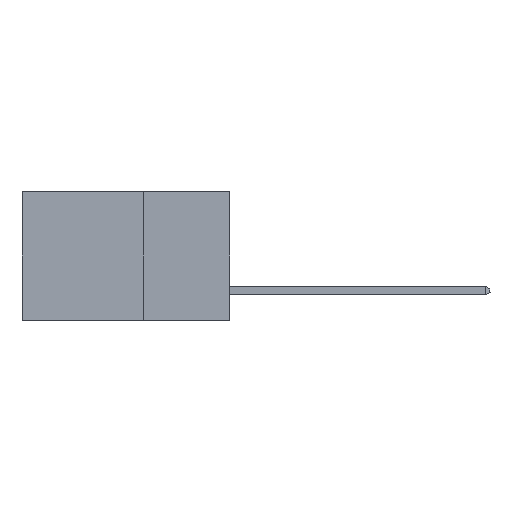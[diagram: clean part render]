
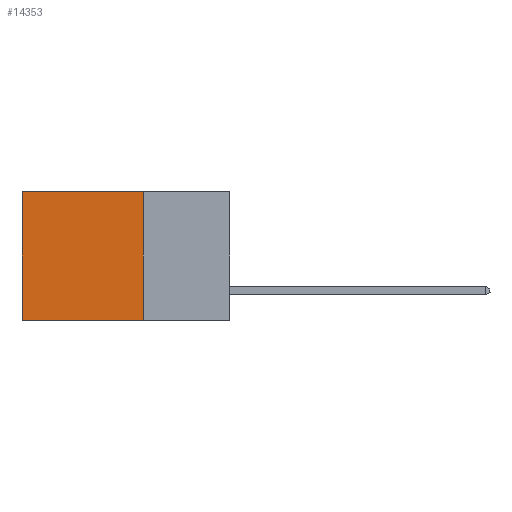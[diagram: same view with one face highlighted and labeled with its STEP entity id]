
A CAD part, left-side view. The second image highlights one B-rep face of the part: STEP entity #14353.
In plain terms, the highlighted planar face has unit normal (-1, 0, 0).
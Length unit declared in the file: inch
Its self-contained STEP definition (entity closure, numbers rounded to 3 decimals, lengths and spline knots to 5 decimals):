
#10 = EDGE_CURVE ( 'NONE', #11506, #3457, #2762, .T. ) ;
#201 = CARTESIAN_POINT ( 'NONE',  ( 0.298, 0.6, 0. ) ) ;
#273 = CARTESIAN_POINT ( 'NONE',  ( 0.298, 0.6, 0. ) ) ;
#905 = DIRECTION ( 'NONE',  ( 1., 0., 0. ) ) ;
#986 = CARTESIAN_POINT ( 'NONE',  ( 0.298, 0.25, 0. ) ) ;
#1171 = VECTOR ( 'NONE', #10612, 39.37008 ) ;
#1216 = ORIENTED_EDGE ( 'NONE', *, *, #4257, .T. ) ;
#1349 = CARTESIAN_POINT ( 'NONE',  ( 0.298, 0.25, -0.37 ) ) ;
#1497 = DIRECTION ( 'NONE',  ( 0., 1., 0. ) ) ;
#2489 = DIRECTION ( 'NONE',  ( 0., 0., -1. ) ) ;
#2616 = LINE ( 'NONE', #5048, #5979 ) ;
#2762 = LINE ( 'NONE', #4733, #1171 ) ;
#3457 = VERTEX_POINT ( 'NONE', #273 ) ;
#4257 = EDGE_CURVE ( 'NONE', #3457, #8376, #6831, .T. ) ;
#4314 = LINE ( 'NONE', #1349, #5175 ) ;
#4332 = VECTOR ( 'NONE', #2489, 39.37008 ) ;
#4733 = CARTESIAN_POINT ( 'NONE',  ( 0.298, 0.25, 0. ) ) ;
#4811 = FACE_OUTER_BOUND ( 'NONE', #7956, .T. ) ;
#5048 = CARTESIAN_POINT ( 'NONE',  ( 0.298, 0.25, 0. ) ) ;
#5175 = VECTOR ( 'NONE', #1497, 39.37008 ) ;
#5849 = VERTEX_POINT ( 'NONE', #9368 ) ;
#5979 = VECTOR ( 'NONE', #6074, 39.37008 ) ;
#6074 = DIRECTION ( 'NONE',  ( 0., 0., -1. ) ) ;
#6831 = LINE ( 'NONE', #201, #4332 ) ;
#7956 = EDGE_LOOP ( 'NONE', ( #1216, #8602, #8027, #11502 ) ) ;
#8027 = ORIENTED_EDGE ( 'NONE', *, *, #12370, .F. ) ;
#8376 = VERTEX_POINT ( 'NONE', #12234 ) ;
#8602 = ORIENTED_EDGE ( 'NONE', *, *, #9770, .F. ) ;
#9368 = CARTESIAN_POINT ( 'NONE',  ( 0.298, 0.25, -0.37 ) ) ;
#9728 = PLANE ( 'NONE',  #12590 ) ;
#9770 = EDGE_CURVE ( 'NONE', #5849, #8376, #4314, .T. ) ;
#9836 = CARTESIAN_POINT ( 'NONE',  ( 0.298, 0.25, 0. ) ) ;
#10612 = DIRECTION ( 'NONE',  ( 0., 1., 0. ) ) ;
#11502 = ORIENTED_EDGE ( 'NONE', *, *, #10, .T. ) ;
#11506 = VERTEX_POINT ( 'NONE', #986 ) ;
#12234 = CARTESIAN_POINT ( 'NONE',  ( 0.298, 0.6, -0.37 ) ) ;
#12370 = EDGE_CURVE ( 'NONE', #11506, #5849, #2616, .T. ) ;
#12590 = AXIS2_PLACEMENT_3D ( 'NONE', #9836, #905, #14529 ) ;
#14353 = ADVANCED_FACE ( 'NONE', ( #4811 ), #9728, .F. ) ;
#14529 = DIRECTION ( 'NONE',  ( 0., 0., -1. ) ) ;
